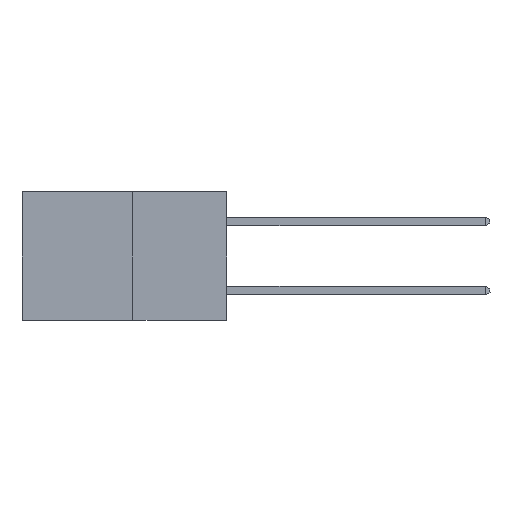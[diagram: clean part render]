
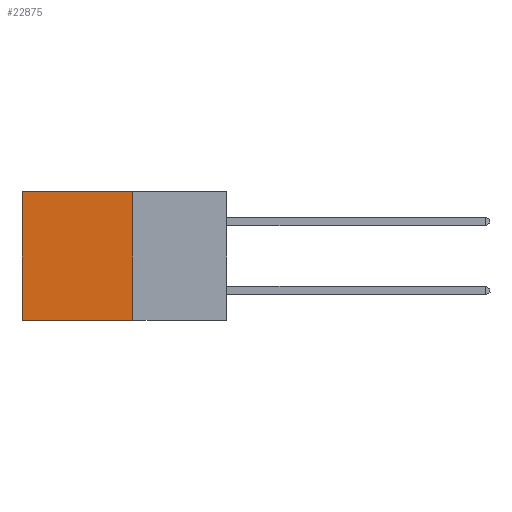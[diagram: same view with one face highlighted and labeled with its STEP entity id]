
A CAD part, left-side view. The second image highlights one B-rep face of the part: STEP entity #22875.
In plain terms, the highlighted planar face has unit normal (-1, 0, 0).
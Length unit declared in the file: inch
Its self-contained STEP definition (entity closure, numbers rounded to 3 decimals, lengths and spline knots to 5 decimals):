
#206 = LINE ( 'NONE', #17978, #11172 ) ;
#713 = CARTESIAN_POINT ( 'NONE',  ( 0.277, 0.27, -0.37 ) ) ;
#957 = CARTESIAN_POINT ( 'NONE',  ( 0.277, 0.59, -0.37 ) ) ;
#2408 = ORIENTED_EDGE ( 'NONE', *, *, #27776, .F. ) ;
#3624 = DIRECTION ( 'NONE',  ( 0., 0., -1. ) ) ;
#4009 = LINE ( 'NONE', #8678, #15467 ) ;
#5640 = LINE ( 'NONE', #713, #26438 ) ;
#6208 = FACE_OUTER_BOUND ( 'NONE', #8376, .T. ) ;
#7270 = DIRECTION ( 'NONE',  ( 0., 1., 0. ) ) ;
#7475 = VERTEX_POINT ( 'NONE', #19203 ) ;
#8376 = EDGE_LOOP ( 'NONE', ( #15866, #11814, #2408, #21783 ) ) ;
#8678 = CARTESIAN_POINT ( 'NONE',  ( 0.277, 0.27, 0. ) ) ;
#8867 = VERTEX_POINT ( 'NONE', #16055 ) ;
#10881 = AXIS2_PLACEMENT_3D ( 'NONE', #16416, #16511, #3624 ) ;
#11172 = VECTOR ( 'NONE', #7270, 39.37008 ) ;
#11814 = ORIENTED_EDGE ( 'NONE', *, *, #12896, .F. ) ;
#12896 = EDGE_CURVE ( 'NONE', #7475, #23487, #206, .T. ) ;
#13417 = EDGE_CURVE ( 'NONE', #20484, #8867, #4009, .T. ) ;
#15467 = VECTOR ( 'NONE', #25826, 39.37008 ) ;
#15588 = CARTESIAN_POINT ( 'NONE',  ( 0.277, 0.59, -0.37 ) ) ;
#15866 = ORIENTED_EDGE ( 'NONE', *, *, #21834, .T. ) ;
#15969 = LINE ( 'NONE', #15588, #21112 ) ;
#16055 = CARTESIAN_POINT ( 'NONE',  ( 0.277, 0.59, 0. ) ) ;
#16416 = CARTESIAN_POINT ( 'NONE',  ( 0.277, 0.27, -0.37 ) ) ;
#16511 = DIRECTION ( 'NONE',  ( 1., 0., 0. ) ) ;
#17771 = DIRECTION ( 'NONE',  ( 0., 0., -1. ) ) ;
#17978 = CARTESIAN_POINT ( 'NONE',  ( 0.277, 0.27, -0.37 ) ) ;
#18088 = DIRECTION ( 'NONE',  ( 0., 0., -1. ) ) ;
#19203 = CARTESIAN_POINT ( 'NONE',  ( 0.277, 0.27, -0.37 ) ) ;
#20484 = VERTEX_POINT ( 'NONE', #26326 ) ;
#21112 = VECTOR ( 'NONE', #17771, 39.37008 ) ;
#21783 = ORIENTED_EDGE ( 'NONE', *, *, #13417, .T. ) ;
#21834 = EDGE_CURVE ( 'NONE', #8867, #23487, #15969, .T. ) ;
#22875 = ADVANCED_FACE ( 'NONE', ( #6208 ), #25109, .F. ) ;
#23487 = VERTEX_POINT ( 'NONE', #957 ) ;
#25109 = PLANE ( 'NONE',  #10881 ) ;
#25826 = DIRECTION ( 'NONE',  ( 0., 1., 0. ) ) ;
#26326 = CARTESIAN_POINT ( 'NONE',  ( 0.277, 0.27, 0. ) ) ;
#26438 = VECTOR ( 'NONE', #18088, 39.37008 ) ;
#27776 = EDGE_CURVE ( 'NONE', #20484, #7475, #5640, .T. ) ;
